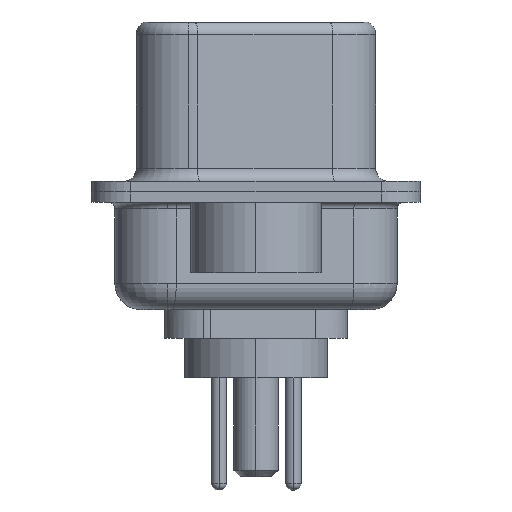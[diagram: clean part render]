
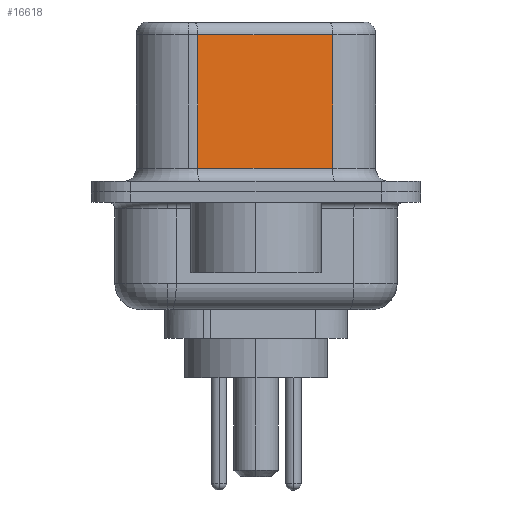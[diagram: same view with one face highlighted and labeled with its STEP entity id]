
A CAD part, left-side view. The second image highlights one B-rep face of the part: STEP entity #16618.
In plain terms, the highlighted planar face has unit normal (-0.985, -0.174, 0).
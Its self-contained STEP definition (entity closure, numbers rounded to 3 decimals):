
#211 = LINE ( 'NONE', #3301, #11112 ) ;
#654 = FACE_OUTER_BOUND ( 'NONE', #14108, .T. ) ;
#1071 = CARTESIAN_POINT ( 'NONE',  ( 3.675, 2.233, 6.02 ) ) ;
#1114 = VERTEX_POINT ( 'NONE', #1071 ) ;
#1219 = PLANE ( 'NONE',  #16147 ) ;
#3145 = LINE ( 'NONE', #8598, #13901 ) ;
#3301 = CARTESIAN_POINT ( 'NONE',  ( 4.585, -2.927, 6.02 ) ) ;
#3889 = DIRECTION ( 'NONE',  ( 0., 0., -1. ) ) ;
#5098 = ORIENTED_EDGE ( 'NONE', *, *, #16738, .F. ) ;
#5488 = VERTEX_POINT ( 'NONE', #17690 ) ;
#5890 = EDGE_CURVE ( 'NONE', #15393, #16940, #10884, .T. ) ;
#6081 = CARTESIAN_POINT ( 'NONE',  ( 4.585, -2.927, 0.9 ) ) ;
#8332 = DIRECTION ( 'NONE',  ( -0.174, 0.985, 0. ) ) ;
#8598 = CARTESIAN_POINT ( 'NONE',  ( 4.585, -2.927, 6.52 ) ) ;
#9452 = CARTESIAN_POINT ( 'NONE',  ( 3.675, 2.233, 6.52 ) ) ;
#9533 = ORIENTED_EDGE ( 'NONE', *, *, #15809, .T. ) ;
#9997 = DIRECTION ( 'NONE',  ( 0., 0., -1. ) ) ;
#10317 = DIRECTION ( 'NONE',  ( -0.174, 0.985, 0. ) ) ;
#10457 = VECTOR ( 'NONE', #12562, 1000. ) ;
#10884 = LINE ( 'NONE', #17440, #10457 ) ;
#11112 = VECTOR ( 'NONE', #10317, 1000. ) ;
#12562 = DIRECTION ( 'NONE',  ( 0.174, -0.985, 0. ) ) ;
#12622 = ORIENTED_EDGE ( 'NONE', *, *, #5890, .T. ) ;
#12889 = CARTESIAN_POINT ( 'NONE',  ( 3.675, 2.233, 0.9 ) ) ;
#13901 = VECTOR ( 'NONE', #9997, 1000. ) ;
#13903 = CARTESIAN_POINT ( 'NONE',  ( 4.585, -2.927, 6.52 ) ) ;
#14108 = EDGE_LOOP ( 'NONE', ( #5098, #16202, #9533, #12622 ) ) ;
#15374 = LINE ( 'NONE', #9452, #18273 ) ;
#15393 = VERTEX_POINT ( 'NONE', #12889 ) ;
#15533 = EDGE_CURVE ( 'NONE', #5488, #1114, #211, .T. ) ;
#15809 = EDGE_CURVE ( 'NONE', #1114, #15393, #15374, .T. ) ;
#16147 = AXIS2_PLACEMENT_3D ( 'NONE', #13903, #16648, #8332 ) ;
#16202 = ORIENTED_EDGE ( 'NONE', *, *, #15533, .T. ) ;
#16618 = ADVANCED_FACE ( 'NONE', ( #654 ), #1219, .F. ) ;
#16648 = DIRECTION ( 'NONE',  ( 0.985, 0.174, 0. ) ) ;
#16738 = EDGE_CURVE ( 'NONE', #5488, #16940, #3145, .T. ) ;
#16940 = VERTEX_POINT ( 'NONE', #6081 ) ;
#17440 = CARTESIAN_POINT ( 'NONE',  ( 4.585, -2.927, 0.9 ) ) ;
#17690 = CARTESIAN_POINT ( 'NONE',  ( 4.585, -2.927, 6.02 ) ) ;
#18273 = VECTOR ( 'NONE', #3889, 1000. ) ;
